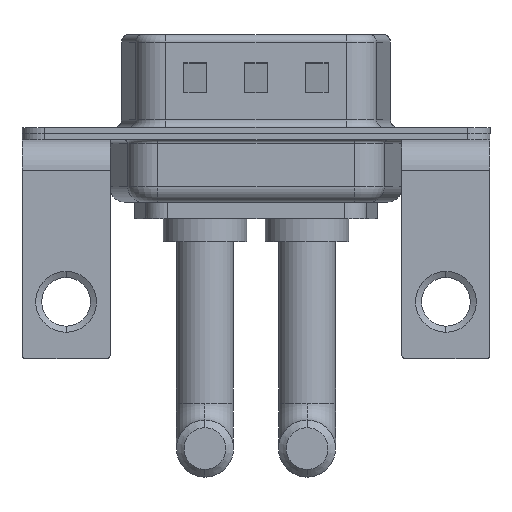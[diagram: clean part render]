
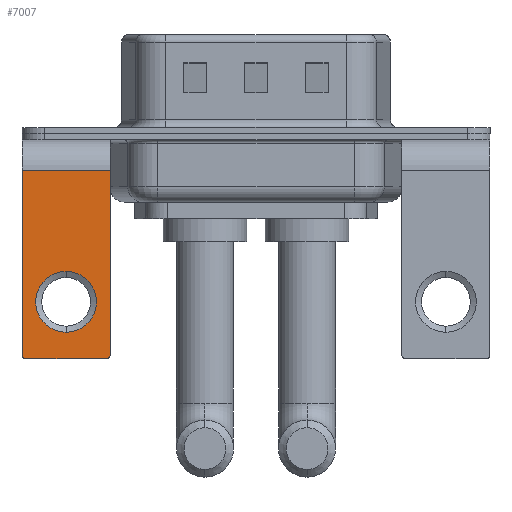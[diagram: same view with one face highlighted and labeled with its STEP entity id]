
A CAD part, front view. The second image highlights one B-rep face of the part: STEP entity #7007.
In plain terms, the highlighted planar face has unit normal (0, -1, 0).
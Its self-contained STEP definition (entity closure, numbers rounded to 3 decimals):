
#286 = DIRECTION ( 'NONE',  ( 0., 0., 1. ) ) ;
#388 = ORIENTED_EDGE ( 'NONE', *, *, #14567, .T. ) ;
#581 = CARTESIAN_POINT ( 'NONE',  ( -2.9, -6.25, -14.55 ) ) ;
#700 = AXIS2_PLACEMENT_3D ( 'NONE', #7231, #11898, #11211 ) ;
#1063 = LINE ( 'NONE', #5756, #14929 ) ;
#1361 = VERTEX_POINT ( 'NONE', #12840 ) ;
#1627 = VERTEX_POINT ( 'NONE', #13737 ) ;
#1749 = ORIENTED_EDGE ( 'NONE', *, *, #11886, .T. ) ;
#1868 = FACE_OUTER_BOUND ( 'NONE', #9982, .T. ) ;
#1893 = VECTOR ( 'NONE', #12381, 1000. ) ;
#2133 = VERTEX_POINT ( 'NONE', #9162 ) ;
#2173 = CARTESIAN_POINT ( 'NONE',  ( 2.65, -6.25, -14.55 ) ) ;
#2411 = ORIENTED_EDGE ( 'NONE', *, *, #6948, .T. ) ;
#2417 = DIRECTION ( 'NONE',  ( 0., 1., 0. ) ) ;
#2563 = CARTESIAN_POINT ( 'NONE',  ( 0., -6.25, -11.07 ) ) ;
#2650 = DIRECTION ( 'NONE',  ( 0., 0., -1. ) ) ;
#2777 = EDGE_CURVE ( 'NONE', #1361, #9314, #8499, .T. ) ;
#3113 = DIRECTION ( 'NONE',  ( 0., -1., 0. ) ) ;
#3289 = CARTESIAN_POINT ( 'NONE',  ( 0., -6.25, -11.07 ) ) ;
#3644 = CARTESIAN_POINT ( 'NONE',  ( -2.9, -6.25, -2.4 ) ) ;
#3673 = CIRCLE ( 'NONE', #6132, 0.25 ) ;
#4942 = EDGE_CURVE ( 'NONE', #13602, #13861, #7803, .T. ) ;
#5113 = CARTESIAN_POINT ( 'NONE',  ( 2.9, -6.25, -2.4 ) ) ;
#5395 = VERTEX_POINT ( 'NONE', #7066 ) ;
#5413 = VECTOR ( 'NONE', #2650, 1000. ) ;
#5429 = DIRECTION ( 'NONE',  ( 0., 0., 1. ) ) ;
#5433 = AXIS2_PLACEMENT_3D ( 'NONE', #3289, #13538, #11487 ) ;
#5465 = DIRECTION ( 'NONE',  ( -1., 0., 0. ) ) ;
#5643 = AXIS2_PLACEMENT_3D ( 'NONE', #5113, #6575, #6346 ) ;
#5663 = ORIENTED_EDGE ( 'NONE', *, *, #9799, .T. ) ;
#5665 = VERTEX_POINT ( 'NONE', #581 ) ;
#5756 = CARTESIAN_POINT ( 'NONE',  ( 2.9, -6.25, -2.4 ) ) ;
#6132 = AXIS2_PLACEMENT_3D ( 'NONE', #2173, #3113, #5429 ) ;
#6272 = EDGE_LOOP ( 'NONE', ( #2411, #5663 ) ) ;
#6346 = DIRECTION ( 'NONE',  ( 0., 0., 1. ) ) ;
#6465 = ORIENTED_EDGE ( 'NONE', *, *, #9379, .T. ) ;
#6575 = DIRECTION ( 'NONE',  ( 0., 1., 0. ) ) ;
#6655 = CARTESIAN_POINT ( 'NONE',  ( 2.9, -6.25, -14.8 ) ) ;
#6948 = EDGE_CURVE ( 'NONE', #1627, #2133, #9308, .T. ) ;
#7007 = ADVANCED_FACE ( 'NONE', ( #12317, #1868 ), #10035, .F. ) ;
#7066 = CARTESIAN_POINT ( 'NONE',  ( -2.9, -6.25, -2.4 ) ) ;
#7098 = AXIS2_PLACEMENT_3D ( 'NONE', #2563, #2417, #286 ) ;
#7231 = CARTESIAN_POINT ( 'NONE',  ( -2.65, -6.25, -14.55 ) ) ;
#7309 = CIRCLE ( 'NONE', #700, 0.25 ) ;
#7803 = LINE ( 'NONE', #6655, #1893 ) ;
#7858 = VECTOR ( 'NONE', #10411, 1000. ) ;
#8269 = CARTESIAN_POINT ( 'NONE',  ( 2.65, -6.25, -14.8 ) ) ;
#8470 = ORIENTED_EDGE ( 'NONE', *, *, #2777, .F. ) ;
#8499 = LINE ( 'NONE', #10872, #5413 ) ;
#8691 = ORIENTED_EDGE ( 'NONE', *, *, #12561, .T. ) ;
#9071 = CARTESIAN_POINT ( 'NONE',  ( 2.9, -6.25, -14.55 ) ) ;
#9162 = CARTESIAN_POINT ( 'NONE',  ( 0., -6.25, -9.07 ) ) ;
#9308 = CIRCLE ( 'NONE', #7098, 2. ) ;
#9314 = VERTEX_POINT ( 'NONE', #9071 ) ;
#9379 = EDGE_CURVE ( 'NONE', #1361, #5395, #1063, .T. ) ;
#9407 = LINE ( 'NONE', #3644, #7858 ) ;
#9799 = EDGE_CURVE ( 'NONE', #2133, #1627, #12023, .T. ) ;
#9982 = EDGE_LOOP ( 'NONE', ( #388, #1749, #11136, #8691, #8470, #6465 ) ) ;
#10035 = PLANE ( 'NONE',  #5643 ) ;
#10411 = DIRECTION ( 'NONE',  ( 0., 0., -1. ) ) ;
#10872 = CARTESIAN_POINT ( 'NONE',  ( 2.9, -6.25, -2.4 ) ) ;
#11136 = ORIENTED_EDGE ( 'NONE', *, *, #4942, .F. ) ;
#11211 = DIRECTION ( 'NONE',  ( 0., 0., 1. ) ) ;
#11487 = DIRECTION ( 'NONE',  ( 0., 0., 1. ) ) ;
#11886 = EDGE_CURVE ( 'NONE', #5665, #13861, #7309, .T. ) ;
#11898 = DIRECTION ( 'NONE',  ( 0., -1., 0. ) ) ;
#12023 = CIRCLE ( 'NONE', #5433, 2. ) ;
#12317 = FACE_BOUND ( 'NONE', #6272, .T. ) ;
#12381 = DIRECTION ( 'NONE',  ( -1., 0., 0. ) ) ;
#12561 = EDGE_CURVE ( 'NONE', #13602, #9314, #3673, .T. ) ;
#12758 = CARTESIAN_POINT ( 'NONE',  ( -2.65, -6.25, -14.8 ) ) ;
#12840 = CARTESIAN_POINT ( 'NONE',  ( 2.9, -6.25, -2.4 ) ) ;
#13538 = DIRECTION ( 'NONE',  ( 0., 1., 0. ) ) ;
#13602 = VERTEX_POINT ( 'NONE', #8269 ) ;
#13737 = CARTESIAN_POINT ( 'NONE',  ( 0., -6.25, -13.07 ) ) ;
#13861 = VERTEX_POINT ( 'NONE', #12758 ) ;
#14567 = EDGE_CURVE ( 'NONE', #5395, #5665, #9407, .T. ) ;
#14929 = VECTOR ( 'NONE', #5465, 1000. ) ;
